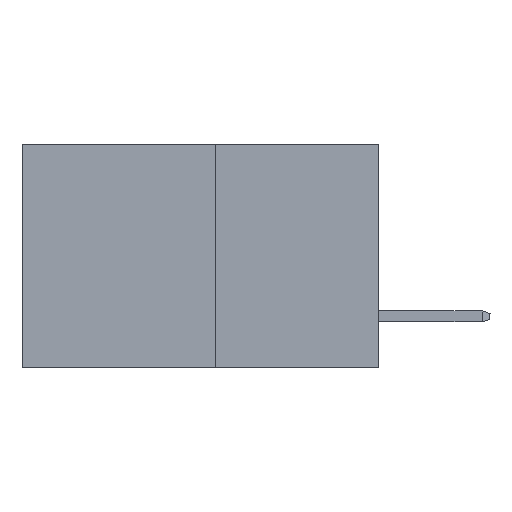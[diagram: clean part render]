
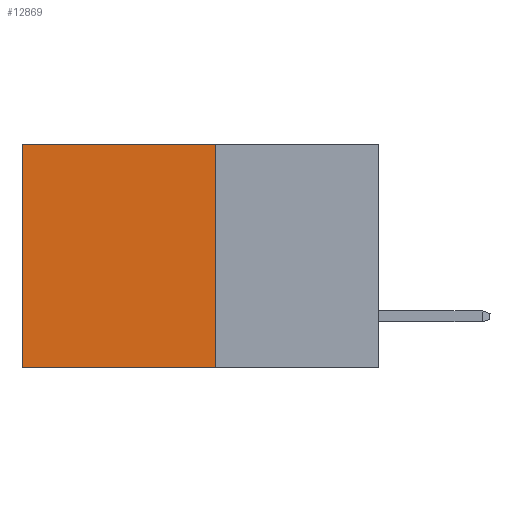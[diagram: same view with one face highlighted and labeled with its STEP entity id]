
A CAD part, left-side view. The second image highlights one B-rep face of the part: STEP entity #12869.
In plain terms, the highlighted planar face has unit normal (-1, 0, 0).
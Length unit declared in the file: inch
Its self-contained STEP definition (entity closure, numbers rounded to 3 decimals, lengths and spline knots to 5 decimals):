
#441 = PLANE ( 'NONE',  #2649 ) ;
#466 = VERTEX_POINT ( 'NONE', #3671 ) ;
#505 = LINE ( 'NONE', #8336, #12236 ) ;
#2188 = CARTESIAN_POINT ( 'NONE',  ( 0.277, 0.27, -0.37 ) ) ;
#2649 = AXIS2_PLACEMENT_3D ( 'NONE', #8628, #9753, #2861 ) ;
#2861 = DIRECTION ( 'NONE',  ( 0., 0., -1. ) ) ;
#2875 = EDGE_CURVE ( 'NONE', #466, #14050, #12588, .T. ) ;
#2955 = LINE ( 'NONE', #11966, #11633 ) ;
#3019 = DIRECTION ( 'NONE',  ( 0., 1., 0. ) ) ;
#3671 = CARTESIAN_POINT ( 'NONE',  ( 0.277, 0.59, 0. ) ) ;
#3740 = VERTEX_POINT ( 'NONE', #2188 ) ;
#3906 = ORIENTED_EDGE ( 'NONE', *, *, #10000, .T. ) ;
#4869 = FACE_OUTER_BOUND ( 'NONE', #9423, .T. ) ;
#6092 = DIRECTION ( 'NONE',  ( 0., 1., 0. ) ) ;
#6727 = VECTOR ( 'NONE', #9653, 39.37008 ) ;
#6838 = VECTOR ( 'NONE', #9540, 39.37008 ) ;
#6873 = CARTESIAN_POINT ( 'NONE',  ( 0.277, 0.27, 0. ) ) ;
#7380 = CARTESIAN_POINT ( 'NONE',  ( 0.277, 0.27, -0.37 ) ) ;
#8336 = CARTESIAN_POINT ( 'NONE',  ( 0.277, 0.27, -0.37 ) ) ;
#8389 = ORIENTED_EDGE ( 'NONE', *, *, #10391, .F. ) ;
#8628 = CARTESIAN_POINT ( 'NONE',  ( 0.277, 0.27, -0.37 ) ) ;
#9049 = ORIENTED_EDGE ( 'NONE', *, *, #13315, .F. ) ;
#9423 = EDGE_LOOP ( 'NONE', ( #14220, #8389, #9049, #3906 ) ) ;
#9540 = DIRECTION ( 'NONE',  ( 0., 0., -1. ) ) ;
#9653 = DIRECTION ( 'NONE',  ( 0., 0., -1. ) ) ;
#9731 = LINE ( 'NONE', #7380, #6727 ) ;
#9753 = DIRECTION ( 'NONE',  ( 1., 0., 0. ) ) ;
#10000 = EDGE_CURVE ( 'NONE', #10730, #466, #2955, .T. ) ;
#10081 = CARTESIAN_POINT ( 'NONE',  ( 0.277, 0.59, -0.37 ) ) ;
#10391 = EDGE_CURVE ( 'NONE', #3740, #14050, #505, .T. ) ;
#10730 = VERTEX_POINT ( 'NONE', #6873 ) ;
#11633 = VECTOR ( 'NONE', #3019, 39.37008 ) ;
#11966 = CARTESIAN_POINT ( 'NONE',  ( 0.277, 0.27, 0. ) ) ;
#12236 = VECTOR ( 'NONE', #6092, 39.37008 ) ;
#12588 = LINE ( 'NONE', #10081, #6838 ) ;
#12636 = CARTESIAN_POINT ( 'NONE',  ( 0.277, 0.59, -0.37 ) ) ;
#12869 = ADVANCED_FACE ( 'NONE', ( #4869 ), #441, .F. ) ;
#13315 = EDGE_CURVE ( 'NONE', #10730, #3740, #9731, .T. ) ;
#14050 = VERTEX_POINT ( 'NONE', #12636 ) ;
#14220 = ORIENTED_EDGE ( 'NONE', *, *, #2875, .T. ) ;
